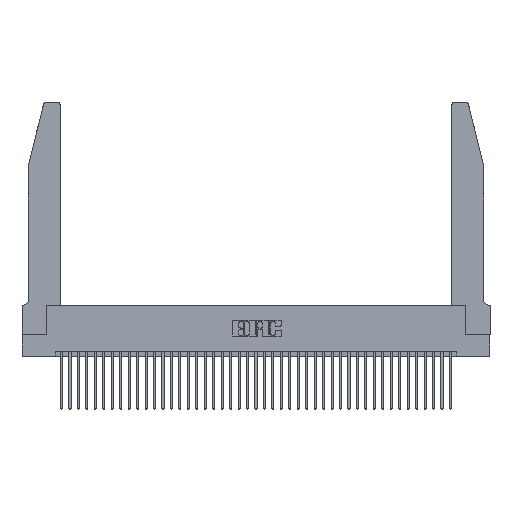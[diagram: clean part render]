
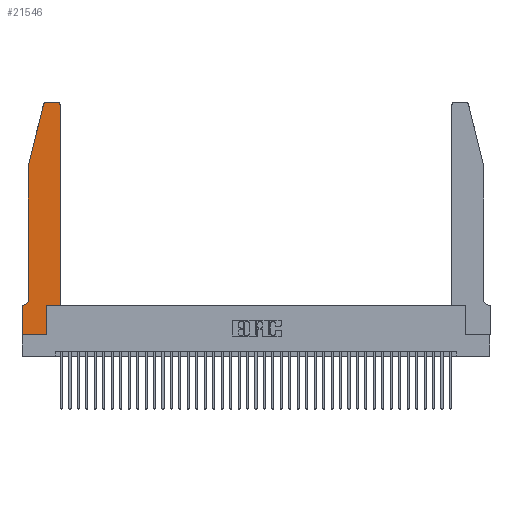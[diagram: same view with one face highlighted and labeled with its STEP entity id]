
A CAD part, top view. The second image highlights one B-rep face of the part: STEP entity #21546.
In plain terms, the highlighted planar face has unit normal (0, 0, 1).
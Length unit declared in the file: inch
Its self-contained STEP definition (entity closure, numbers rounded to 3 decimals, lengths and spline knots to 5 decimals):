
#468 = DIRECTION ( 'NONE',  ( 0., 0., 1. ) ) ;
#847 = VERTEX_POINT ( 'NONE', #24263 ) ;
#993 = LINE ( 'NONE', #21141, #33698 ) ;
#1297 = DIRECTION ( 'NONE',  ( 0., 1., 0. ) ) ;
#3112 = LINE ( 'NONE', #11796, #35738 ) ;
#4081 = DIRECTION ( 'NONE',  ( 0., 0., -1. ) ) ;
#4283 = EDGE_CURVE ( 'NONE', #35122, #27363, #38050, .T. ) ;
#4512 = CARTESIAN_POINT ( 'NONE',  ( 0.0055, 0.42, 0.37 ) ) ;
#5658 = AXIS2_PLACEMENT_3D ( 'NONE', #28038, #21781, #30064 ) ;
#5723 = ORIENTED_EDGE ( 'NONE', *, *, #23978, .T. ) ;
#6005 = LINE ( 'NONE', #34226, #21317 ) ;
#6965 = DIRECTION ( 'NONE',  ( -1., 0., 0. ) ) ;
#7235 = ORIENTED_EDGE ( 'NONE', *, *, #35168, .T. ) ;
#7541 = CARTESIAN_POINT ( 'NONE',  ( 0.0755, 2., 0.37 ) ) ;
#7712 = ORIENTED_EDGE ( 'NONE', *, *, #31798, .T. ) ;
#7853 = VECTOR ( 'NONE', #34647, 39.37008 ) ;
#7983 = VERTEX_POINT ( 'NONE', #21681 ) ;
#8258 = VECTOR ( 'NONE', #25917, 39.37008 ) ;
#8793 = AXIS2_PLACEMENT_3D ( 'NONE', #4512, #4081, #19947 ) ;
#9405 = ORIENTED_EDGE ( 'NONE', *, *, #33952, .T. ) ;
#10871 = CARTESIAN_POINT ( 'NONE',  ( 0., 0., 0.37 ) ) ;
#10996 = DIRECTION ( 'NONE',  ( 0., -1., 0. ) ) ;
#11796 = CARTESIAN_POINT ( 'NONE',  ( 0.4505, 0.35, 0.37 ) ) ;
#12164 = EDGE_CURVE ( 'NONE', #7983, #22448, #25707, .T. ) ;
#12412 = CARTESIAN_POINT ( 'NONE',  ( 0.4505, 0.35, 0.37 ) ) ;
#13587 = VERTEX_POINT ( 'NONE', #20310 ) ;
#14184 = ORIENTED_EDGE ( 'NONE', *, *, #33719, .T. ) ;
#15292 = LINE ( 'NONE', #10871, #36047 ) ;
#15322 = VECTOR ( 'NONE', #6965, 39.37008 ) ;
#15895 = ORIENTED_EDGE ( 'NONE', *, *, #32197, .T. ) ;
#17658 = VERTEX_POINT ( 'NONE', #35105 ) ;
#18157 = CARTESIAN_POINT ( 'NONE',  ( 0., 0., 0.37 ) ) ;
#18300 = DIRECTION ( 'NONE',  ( 0., -1., 0. ) ) ;
#18312 = DIRECTION ( 'NONE',  ( 1., 0., 0. ) ) ;
#18645 = PLANE ( 'NONE',  #5658 ) ;
#19301 = CARTESIAN_POINT ( 'NONE',  ( 0.0755, 0.35, 0.37 ) ) ;
#19486 = ORIENTED_EDGE ( 'NONE', *, *, #12164, .T. ) ;
#19947 = DIRECTION ( 'NONE',  ( -1., 0., 0. ) ) ;
#20113 = VERTEX_POINT ( 'NONE', #26144 ) ;
#20310 = CARTESIAN_POINT ( 'NONE',  ( 0.25487, 2.72718, 0.37 ) ) ;
#21141 = CARTESIAN_POINT ( 'NONE',  ( 0.0755, 2., 0.37 ) ) ;
#21156 = VECTOR ( 'NONE', #1297, 39.37008 ) ;
#21317 = VECTOR ( 'NONE', #18300, 39.37008 ) ;
#21546 = ADVANCED_FACE ( 'NONE', ( #27214 ), #18645, .T. ) ;
#21681 = CARTESIAN_POINT ( 'NONE',  ( 0., 0., 0.37 ) ) ;
#21781 = DIRECTION ( 'NONE',  ( 0., 0., 1. ) ) ;
#21871 = ORIENTED_EDGE ( 'NONE', *, *, #38631, .T. ) ;
#22141 = EDGE_LOOP ( 'NONE', ( #7235, #5723, #21871, #28308, #15895, #14184, #32435, #19486, #9405, #33359, #7712, #33434 ) ) ;
#22448 = VERTEX_POINT ( 'NONE', #25085 ) ;
#22593 = DIRECTION ( 'NONE',  ( 1., 0., 0. ) ) ;
#22861 = CARTESIAN_POINT ( 'NONE',  ( 0., 0.35, 0.37 ) ) ;
#23382 = CARTESIAN_POINT ( 'NONE',  ( 0.2865, 0.35, 0.37 ) ) ;
#23978 = EDGE_CURVE ( 'NONE', #847, #13587, #25110, .T. ) ;
#24109 = LINE ( 'NONE', #23382, #21156 ) ;
#24263 = CARTESIAN_POINT ( 'NONE',  ( 0.284, 2.75, 0.37 ) ) ;
#24380 = CARTESIAN_POINT ( 'NONE',  ( 0.4205, 2.75, 0.37 ) ) ;
#25085 = CARTESIAN_POINT ( 'NONE',  ( 0.2865, 0., 0.37 ) ) ;
#25110 = CIRCLE ( 'NONE', #32698, 0.03 ) ;
#25642 = CARTESIAN_POINT ( 'NONE',  ( 0.284, 2.72, 0.37 ) ) ;
#25707 = LINE ( 'NONE', #18157, #32637 ) ;
#25780 = CARTESIAN_POINT ( 'NONE',  ( 0.2605, 2.75, 0.37 ) ) ;
#25813 = VERTEX_POINT ( 'NONE', #22861 ) ;
#25917 = DIRECTION ( 'NONE',  ( -1., 0., 0. ) ) ;
#26144 = CARTESIAN_POINT ( 'NONE',  ( 0.0755, 0.42, 0.37 ) ) ;
#26987 = VERTEX_POINT ( 'NONE', #7541 ) ;
#27129 = CARTESIAN_POINT ( 'NONE',  ( 0.0055, 0.35, 0.37 ) ) ;
#27214 = FACE_OUTER_BOUND ( 'NONE', #22141, .T. ) ;
#27363 = VERTEX_POINT ( 'NONE', #24380 ) ;
#28038 = CARTESIAN_POINT ( 'NONE',  ( 0., 0.35, 0.37 ) ) ;
#28308 = ORIENTED_EDGE ( 'NONE', *, *, #32264, .T. ) ;
#28720 = CIRCLE ( 'NONE', #8793, 0.07 ) ;
#29598 = LINE ( 'NONE', #19301, #15322 ) ;
#30064 = DIRECTION ( 'NONE',  ( 1., 0., 0. ) ) ;
#30709 = DIRECTION ( 'NONE',  ( 1., 0., 0. ) ) ;
#30829 = DIRECTION ( 'NONE',  ( 0., 1., 0. ) ) ;
#31798 = EDGE_CURVE ( 'NONE', #39997, #35122, #3112, .T. ) ;
#32197 = EDGE_CURVE ( 'NONE', #20113, #34096, #28720, .T. ) ;
#32264 = EDGE_CURVE ( 'NONE', #26987, #20113, #6005, .T. ) ;
#32435 = ORIENTED_EDGE ( 'NONE', *, *, #40978, .T. ) ;
#32454 = CARTESIAN_POINT ( 'NONE',  ( 0.4505, 2.72, 0.37 ) ) ;
#32637 = VECTOR ( 'NONE', #30709, 39.37008 ) ;
#32698 = AXIS2_PLACEMENT_3D ( 'NONE', #25642, #468, #22593 ) ;
#33359 = ORIENTED_EDGE ( 'NONE', *, *, #34317, .T. ) ;
#33410 = DIRECTION ( 'NONE',  ( 0., 0., 1. ) ) ;
#33434 = ORIENTED_EDGE ( 'NONE', *, *, #4283, .T. ) ;
#33698 = VECTOR ( 'NONE', #38297, 39.37008 ) ;
#33719 = EDGE_CURVE ( 'NONE', #34096, #25813, #29598, .T. ) ;
#33952 = EDGE_CURVE ( 'NONE', #22448, #17658, #24109, .T. ) ;
#34096 = VERTEX_POINT ( 'NONE', #27129 ) ;
#34226 = CARTESIAN_POINT ( 'NONE',  ( 0.0755, 2., 0.37 ) ) ;
#34317 = EDGE_CURVE ( 'NONE', #17658, #39997, #39554, .T. ) ;
#34320 = AXIS2_PLACEMENT_3D ( 'NONE', #36291, #33410, #18312 ) ;
#34647 = DIRECTION ( 'NONE',  ( 1., 0., 0. ) ) ;
#35105 = CARTESIAN_POINT ( 'NONE',  ( 0.2865, 0.35, 0.37 ) ) ;
#35122 = VERTEX_POINT ( 'NONE', #32454 ) ;
#35168 = EDGE_CURVE ( 'NONE', #27363, #847, #38499, .T. ) ;
#35738 = VECTOR ( 'NONE', #30829, 39.37008 ) ;
#36047 = VECTOR ( 'NONE', #10996, 39.37008 ) ;
#36291 = CARTESIAN_POINT ( 'NONE',  ( 0.4205, 2.72, 0.37 ) ) ;
#38050 = CIRCLE ( 'NONE', #34320, 0.03 ) ;
#38297 = DIRECTION ( 'NONE',  ( -0.239, -0.971, 0. ) ) ;
#38499 = LINE ( 'NONE', #25780, #8258 ) ;
#38631 = EDGE_CURVE ( 'NONE', #13587, #26987, #993, .T. ) ;
#39554 = LINE ( 'NONE', #12412, #7853 ) ;
#39997 = VERTEX_POINT ( 'NONE', #40196 ) ;
#40196 = CARTESIAN_POINT ( 'NONE',  ( 0.4505, 0.35, 0.37 ) ) ;
#40978 = EDGE_CURVE ( 'NONE', #25813, #7983, #15292, .T. ) ;
